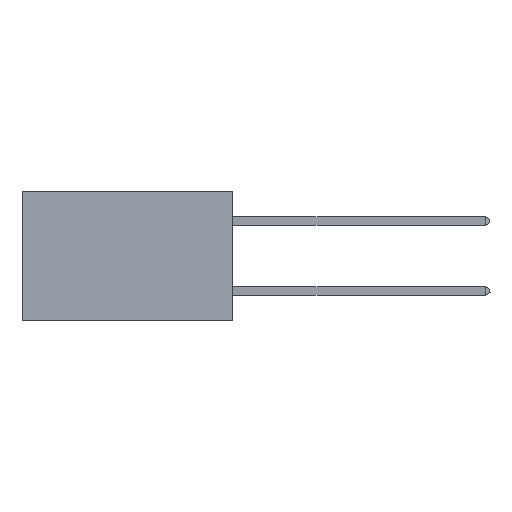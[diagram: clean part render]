
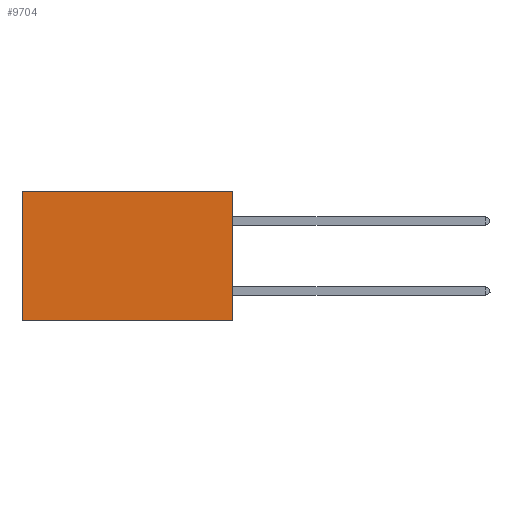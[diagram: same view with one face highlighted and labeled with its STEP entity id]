
A CAD part, left-side view. The second image highlights one B-rep face of the part: STEP entity #9704.
In plain terms, the highlighted planar face has unit normal (-1, 0, 0).
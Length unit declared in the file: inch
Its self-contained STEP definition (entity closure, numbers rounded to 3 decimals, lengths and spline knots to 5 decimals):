
#374 = ORIENTED_EDGE ( 'NONE', *, *, #24862, .F. ) ;
#1471 = CARTESIAN_POINT ( 'NONE',  ( 0.2875, 0., 0. ) ) ;
#1592 = DIRECTION ( 'NONE',  ( 1., 0., 0. ) ) ;
#2431 = DIRECTION ( 'NONE',  ( 0., 0., -1. ) ) ;
#3749 = VECTOR ( 'NONE', #34809, 39.37008 ) ;
#4500 = DIRECTION ( 'NONE',  ( 0., 1., 0. ) ) ;
#4664 = LINE ( 'NONE', #6141, #34874 ) ;
#5416 = VERTEX_POINT ( 'NONE', #7618 ) ;
#6053 = ORIENTED_EDGE ( 'NONE', *, *, #12265, .T. ) ;
#6141 = CARTESIAN_POINT ( 'NONE',  ( 0.2875, 0.6, 0. ) ) ;
#7618 = CARTESIAN_POINT ( 'NONE',  ( 0.2875, 0., 0. ) ) ;
#8754 = DIRECTION ( 'NONE',  ( 0., 1., 0. ) ) ;
#9704 = ADVANCED_FACE ( 'NONE', ( #29662 ), #30857, .F. ) ;
#11286 = EDGE_LOOP ( 'NONE', ( #6053, #18687, #374, #37351 ) ) ;
#11425 = CARTESIAN_POINT ( 'NONE',  ( 0.2875, 0., -0.37 ) ) ;
#12175 = VERTEX_POINT ( 'NONE', #22486 ) ;
#12265 = EDGE_CURVE ( 'NONE', #12175, #18069, #4664, .T. ) ;
#12789 = CARTESIAN_POINT ( 'NONE',  ( 0.2875, 0., -0.37 ) ) ;
#18069 = VERTEX_POINT ( 'NONE', #28532 ) ;
#18687 = ORIENTED_EDGE ( 'NONE', *, *, #29109, .F. ) ;
#19167 = VERTEX_POINT ( 'NONE', #12789 ) ;
#19359 = LINE ( 'NONE', #31553, #3749 ) ;
#19825 = EDGE_CURVE ( 'NONE', #5416, #12175, #23412, .T. ) ;
#20441 = LINE ( 'NONE', #11425, #24140 ) ;
#22069 = CARTESIAN_POINT ( 'NONE',  ( 0.2875, 0., 0. ) ) ;
#22486 = CARTESIAN_POINT ( 'NONE',  ( 0.2875, 0.6, 0. ) ) ;
#23412 = LINE ( 'NONE', #22069, #29846 ) ;
#24140 = VECTOR ( 'NONE', #8754, 39.37008 ) ;
#24862 = EDGE_CURVE ( 'NONE', #5416, #19167, #19359, .T. ) ;
#26695 = DIRECTION ( 'NONE',  ( 0., 0., -1. ) ) ;
#28532 = CARTESIAN_POINT ( 'NONE',  ( 0.2875, 0.6, -0.37 ) ) ;
#29109 = EDGE_CURVE ( 'NONE', #19167, #18069, #20441, .T. ) ;
#29662 = FACE_OUTER_BOUND ( 'NONE', #11286, .T. ) ;
#29846 = VECTOR ( 'NONE', #4500, 39.37008 ) ;
#30857 = PLANE ( 'NONE',  #34399 ) ;
#31553 = CARTESIAN_POINT ( 'NONE',  ( 0.2875, 0., 0. ) ) ;
#34399 = AXIS2_PLACEMENT_3D ( 'NONE', #1471, #1592, #2431 ) ;
#34809 = DIRECTION ( 'NONE',  ( 0., 0., -1. ) ) ;
#34874 = VECTOR ( 'NONE', #26695, 39.37008 ) ;
#37351 = ORIENTED_EDGE ( 'NONE', *, *, #19825, .T. ) ;
